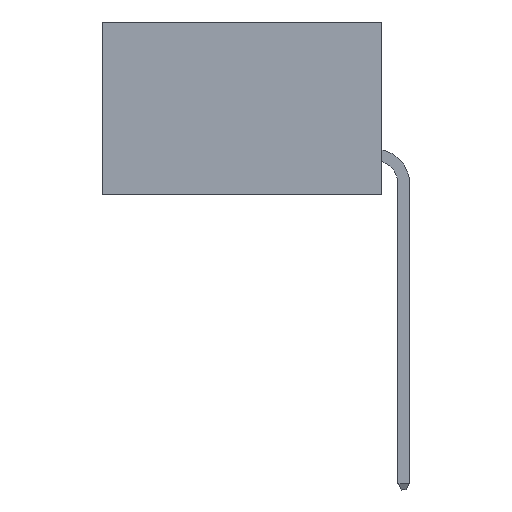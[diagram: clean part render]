
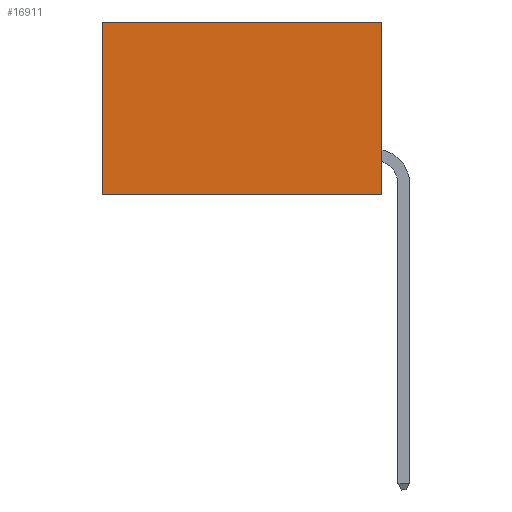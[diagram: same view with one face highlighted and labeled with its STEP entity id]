
A CAD part, left-side view. The second image highlights one B-rep face of the part: STEP entity #16911.
In plain terms, the highlighted planar face has unit normal (-1, 0, 0).
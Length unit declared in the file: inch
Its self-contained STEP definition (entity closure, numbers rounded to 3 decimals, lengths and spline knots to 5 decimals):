
#563 = AXIS2_PLACEMENT_3D ( 'NONE', #16188, #7809, #17558 ) ;
#767 = ORIENTED_EDGE ( 'NONE', *, *, #8584, .T. ) ;
#2133 = EDGE_CURVE ( 'NONE', #13078, #12069, #4449, .T. ) ;
#2889 = CARTESIAN_POINT ( 'NONE',  ( 0.2875, 0., 0. ) ) ;
#3041 = CARTESIAN_POINT ( 'NONE',  ( 0.2875, 0., 0. ) ) ;
#3245 = VECTOR ( 'NONE', #5818, 39.37008 ) ;
#4358 = CARTESIAN_POINT ( 'NONE',  ( 0.2875, 0., -0.37 ) ) ;
#4449 = LINE ( 'NONE', #11525, #10758 ) ;
#4490 = DIRECTION ( 'NONE',  ( 0., 1., 0. ) ) ;
#4816 = DIRECTION ( 'NONE',  ( 0., 0., -1. ) ) ;
#4923 = PLANE ( 'NONE',  #563 ) ;
#5250 = VECTOR ( 'NONE', #5356, 39.37008 ) ;
#5356 = DIRECTION ( 'NONE',  ( 0., 0., -1. ) ) ;
#5818 = DIRECTION ( 'NONE',  ( 0., 1., 0. ) ) ;
#6833 = LINE ( 'NONE', #3041, #13911 ) ;
#7006 = VERTEX_POINT ( 'NONE', #10205 ) ;
#7809 = DIRECTION ( 'NONE',  ( 1., 0., 0. ) ) ;
#8584 = EDGE_CURVE ( 'NONE', #10202, #7006, #12834, .T. ) ;
#9222 = EDGE_CURVE ( 'NONE', #13078, #10202, #6833, .T. ) ;
#10202 = VERTEX_POINT ( 'NONE', #18091 ) ;
#10205 = CARTESIAN_POINT ( 'NONE',  ( 0.2875, 0.6, -0.37 ) ) ;
#10758 = VECTOR ( 'NONE', #4816, 39.37008 ) ;
#10818 = FACE_OUTER_BOUND ( 'NONE', #15826, .T. ) ;
#11525 = CARTESIAN_POINT ( 'NONE',  ( 0.2875, 0., 0. ) ) ;
#12069 = VERTEX_POINT ( 'NONE', #15685 ) ;
#12834 = LINE ( 'NONE', #16611, #5250 ) ;
#12915 = ORIENTED_EDGE ( 'NONE', *, *, #2133, .F. ) ;
#13078 = VERTEX_POINT ( 'NONE', #2889 ) ;
#13911 = VECTOR ( 'NONE', #4490, 39.37008 ) ;
#14922 = EDGE_CURVE ( 'NONE', #12069, #7006, #17781, .T. ) ;
#15237 = ORIENTED_EDGE ( 'NONE', *, *, #14922, .F. ) ;
#15685 = CARTESIAN_POINT ( 'NONE',  ( 0.2875, 0., -0.37 ) ) ;
#15826 = EDGE_LOOP ( 'NONE', ( #767, #15237, #12915, #18403 ) ) ;
#16188 = CARTESIAN_POINT ( 'NONE',  ( 0.2875, 0., 0. ) ) ;
#16611 = CARTESIAN_POINT ( 'NONE',  ( 0.2875, 0.6, 0. ) ) ;
#16911 = ADVANCED_FACE ( 'NONE', ( #10818 ), #4923, .F. ) ;
#17558 = DIRECTION ( 'NONE',  ( 0., 0., -1. ) ) ;
#17781 = LINE ( 'NONE', #4358, #3245 ) ;
#18091 = CARTESIAN_POINT ( 'NONE',  ( 0.2875, 0.6, 0. ) ) ;
#18403 = ORIENTED_EDGE ( 'NONE', *, *, #9222, .T. ) ;
